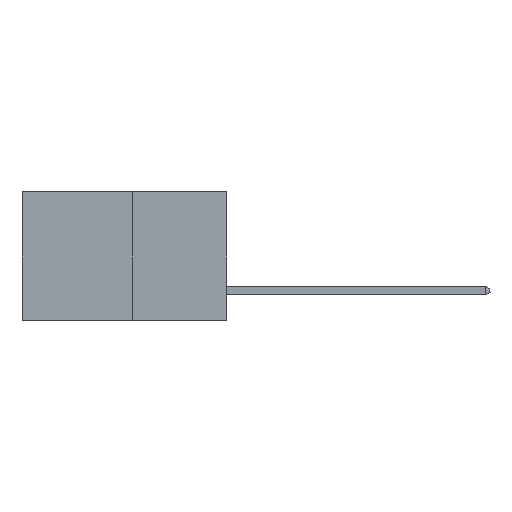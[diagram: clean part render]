
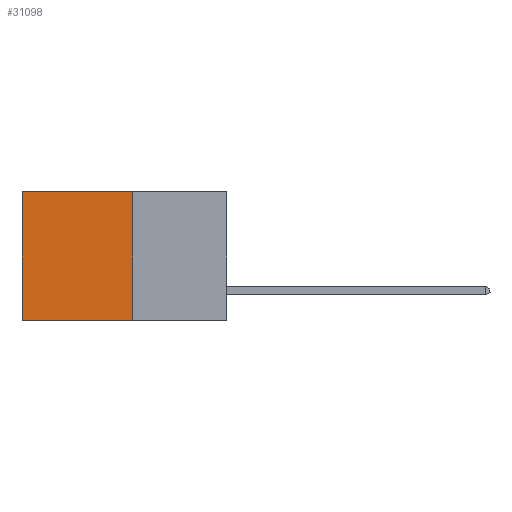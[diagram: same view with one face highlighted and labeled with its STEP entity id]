
A CAD part, left-side view. The second image highlights one B-rep face of the part: STEP entity #31098.
In plain terms, the highlighted planar face has unit normal (-1, 0, 0).
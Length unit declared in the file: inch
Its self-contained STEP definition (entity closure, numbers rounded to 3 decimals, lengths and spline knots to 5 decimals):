
#590 = EDGE_CURVE ( 'NONE', #7825, #14353, #17405, .T. ) ;
#2319 = ORIENTED_EDGE ( 'NONE', *, *, #29243, .F. ) ;
#2933 = AXIS2_PLACEMENT_3D ( 'NONE', #5184, #17677, #27707 ) ;
#3089 = EDGE_CURVE ( 'NONE', #6988, #14353, #8475, .T. ) ;
#4125 = LINE ( 'NONE', #24822, #29894 ) ;
#4349 = CARTESIAN_POINT ( 'NONE',  ( 0.277, 0.27, 0. ) ) ;
#5136 = CARTESIAN_POINT ( 'NONE',  ( 0.277, 0.59, -0.37 ) ) ;
#5184 = CARTESIAN_POINT ( 'NONE',  ( 0.277, 0.27, -0.37 ) ) ;
#6988 = VERTEX_POINT ( 'NONE', #7447 ) ;
#7339 = DIRECTION ( 'NONE',  ( 0., 0., -1. ) ) ;
#7410 = VERTEX_POINT ( 'NONE', #4349 ) ;
#7447 = CARTESIAN_POINT ( 'NONE',  ( 0.277, 0.59, 0. ) ) ;
#7825 = VERTEX_POINT ( 'NONE', #13366 ) ;
#8475 = LINE ( 'NONE', #23706, #29897 ) ;
#9301 = CARTESIAN_POINT ( 'NONE',  ( 0.277, 0.27, 0. ) ) ;
#11853 = DIRECTION ( 'NONE',  ( 0., 1., 0. ) ) ;
#12989 = EDGE_LOOP ( 'NONE', ( #28546, #31479, #2319, #21776 ) ) ;
#13366 = CARTESIAN_POINT ( 'NONE',  ( 0.277, 0.27, -0.37 ) ) ;
#13948 = LINE ( 'NONE', #9301, #25611 ) ;
#14353 = VERTEX_POINT ( 'NONE', #5136 ) ;
#15882 = VECTOR ( 'NONE', #20088, 39.37008 ) ;
#17405 = LINE ( 'NONE', #18771, #15882 ) ;
#17677 = DIRECTION ( 'NONE',  ( 1., 0., 0. ) ) ;
#18771 = CARTESIAN_POINT ( 'NONE',  ( 0.277, 0.27, -0.37 ) ) ;
#20088 = DIRECTION ( 'NONE',  ( 0., 1., 0. ) ) ;
#21776 = ORIENTED_EDGE ( 'NONE', *, *, #24319, .T. ) ;
#23672 = DIRECTION ( 'NONE',  ( 0., 0., -1. ) ) ;
#23706 = CARTESIAN_POINT ( 'NONE',  ( 0.277, 0.59, -0.37 ) ) ;
#24319 = EDGE_CURVE ( 'NONE', #7410, #6988, #13948, .T. ) ;
#24822 = CARTESIAN_POINT ( 'NONE',  ( 0.277, 0.27, -0.37 ) ) ;
#25209 = PLANE ( 'NONE',  #2933 ) ;
#25611 = VECTOR ( 'NONE', #11853, 39.37008 ) ;
#26989 = FACE_OUTER_BOUND ( 'NONE', #12989, .T. ) ;
#27707 = DIRECTION ( 'NONE',  ( 0., 0., -1. ) ) ;
#28546 = ORIENTED_EDGE ( 'NONE', *, *, #3089, .T. ) ;
#29243 = EDGE_CURVE ( 'NONE', #7410, #7825, #4125, .T. ) ;
#29894 = VECTOR ( 'NONE', #7339, 39.37008 ) ;
#29897 = VECTOR ( 'NONE', #23672, 39.37008 ) ;
#31098 = ADVANCED_FACE ( 'NONE', ( #26989 ), #25209, .F. ) ;
#31479 = ORIENTED_EDGE ( 'NONE', *, *, #590, .F. ) ;
